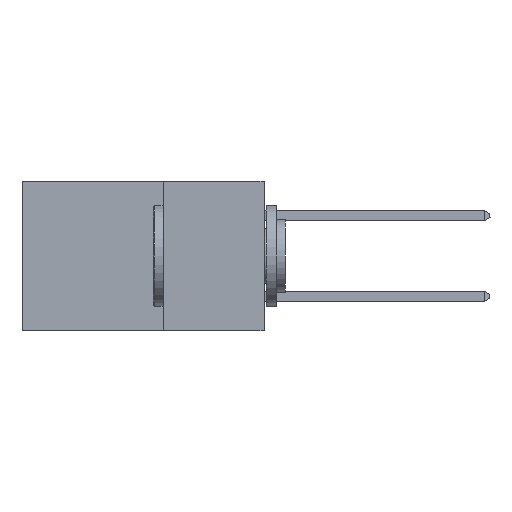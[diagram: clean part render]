
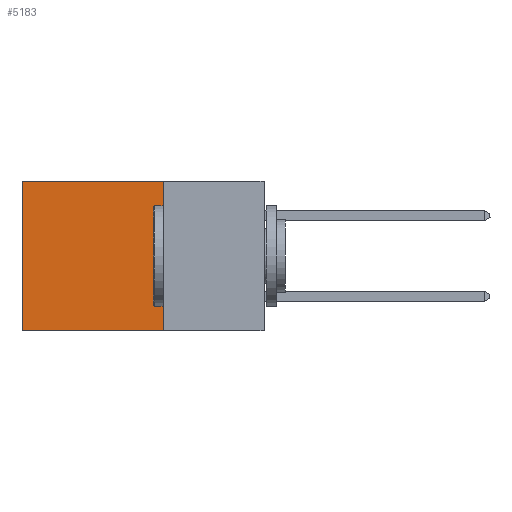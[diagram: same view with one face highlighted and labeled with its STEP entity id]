
A CAD part, left-side view. The second image highlights one B-rep face of the part: STEP entity #5183.
In plain terms, the highlighted planar face has unit normal (-1, 0, 0).
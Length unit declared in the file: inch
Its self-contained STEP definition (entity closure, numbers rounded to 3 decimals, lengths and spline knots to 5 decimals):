
#737 = CARTESIAN_POINT ( 'NONE',  ( 0.298, 0.25, 0. ) ) ;
#781 = FACE_OUTER_BOUND ( 'NONE', #2182, .T. ) ;
#946 = EDGE_CURVE ( 'NONE', #6810, #13011, #9064, .T. ) ;
#1696 = VECTOR ( 'NONE', #5043, 39.37008 ) ;
#1831 = VECTOR ( 'NONE', #3607, 39.37008 ) ;
#1971 = CARTESIAN_POINT ( 'NONE',  ( 0.298, 0.25, -0.37 ) ) ;
#2182 = EDGE_LOOP ( 'NONE', ( #6038, #10511, #10964, #3574 ) ) ;
#2335 = CARTESIAN_POINT ( 'NONE',  ( 0.298, 0.25, 0. ) ) ;
#2553 = CARTESIAN_POINT ( 'NONE',  ( 0.298, 0.6, 0. ) ) ;
#3574 = ORIENTED_EDGE ( 'NONE', *, *, #3813, .T. ) ;
#3607 = DIRECTION ( 'NONE',  ( 0., 0., -1. ) ) ;
#3813 = EDGE_CURVE ( 'NONE', #10102, #8537, #5621, .T. ) ;
#5010 = DIRECTION ( 'NONE',  ( 1., 0., 0. ) ) ;
#5043 = DIRECTION ( 'NONE',  ( 0., 1., 0. ) ) ;
#5183 = ADVANCED_FACE ( 'NONE', ( #781 ), #7110, .F. ) ;
#5607 = CARTESIAN_POINT ( 'NONE',  ( 0.298, 0.25, 0. ) ) ;
#5616 = AXIS2_PLACEMENT_3D ( 'NONE', #737, #5010, #12501 ) ;
#5621 = LINE ( 'NONE', #2335, #10512 ) ;
#5694 = CARTESIAN_POINT ( 'NONE',  ( 0.298, 0.25, 0. ) ) ;
#6038 = ORIENTED_EDGE ( 'NONE', *, *, #12946, .T. ) ;
#6714 = DIRECTION ( 'NONE',  ( 0., 0., -1. ) ) ;
#6810 = VERTEX_POINT ( 'NONE', #1971 ) ;
#7110 = PLANE ( 'NONE',  #5616 ) ;
#7554 = CARTESIAN_POINT ( 'NONE',  ( 0.298, 0.6, -0.37 ) ) ;
#8537 = VERTEX_POINT ( 'NONE', #9931 ) ;
#9064 = LINE ( 'NONE', #11340, #1696 ) ;
#9815 = DIRECTION ( 'NONE',  ( 0., 1., 0. ) ) ;
#9931 = CARTESIAN_POINT ( 'NONE',  ( 0.298, 0.6, 0. ) ) ;
#10102 = VERTEX_POINT ( 'NONE', #5694 ) ;
#10511 = ORIENTED_EDGE ( 'NONE', *, *, #946, .F. ) ;
#10512 = VECTOR ( 'NONE', #9815, 39.37008 ) ;
#10964 = ORIENTED_EDGE ( 'NONE', *, *, #13191, .F. ) ;
#11048 = LINE ( 'NONE', #2553, #1831 ) ;
#11340 = CARTESIAN_POINT ( 'NONE',  ( 0.298, 0.25, -0.37 ) ) ;
#11375 = LINE ( 'NONE', #5607, #13547 ) ;
#12501 = DIRECTION ( 'NONE',  ( 0., 0., -1. ) ) ;
#12946 = EDGE_CURVE ( 'NONE', #8537, #13011, #11048, .T. ) ;
#13011 = VERTEX_POINT ( 'NONE', #7554 ) ;
#13191 = EDGE_CURVE ( 'NONE', #10102, #6810, #11375, .T. ) ;
#13547 = VECTOR ( 'NONE', #6714, 39.37008 ) ;
